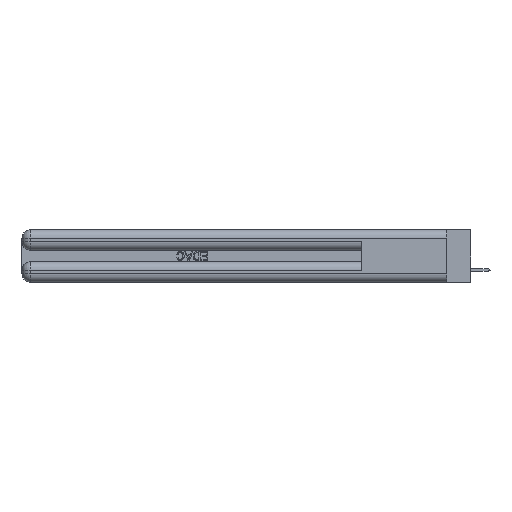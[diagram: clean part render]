
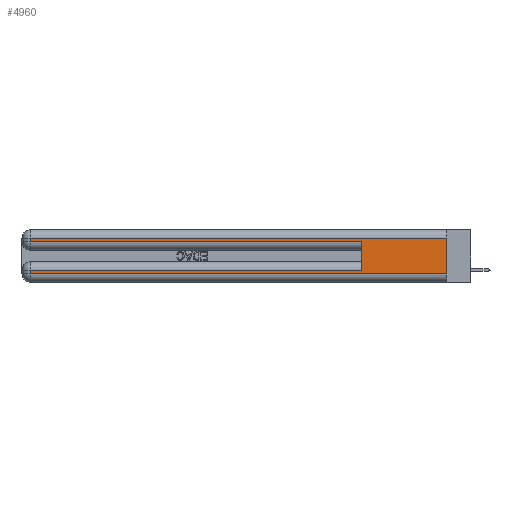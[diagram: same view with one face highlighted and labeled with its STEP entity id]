
A CAD part, left-side view. The second image highlights one B-rep face of the part: STEP entity #4960.
In plain terms, the highlighted planar face has unit normal (-1, 0, 0).
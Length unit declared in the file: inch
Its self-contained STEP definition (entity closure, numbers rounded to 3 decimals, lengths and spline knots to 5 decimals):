
#473 = CARTESIAN_POINT ( 'NONE',  ( 0., 0., 0.06 ) ) ;
#1075 = CARTESIAN_POINT ( 'NONE',  ( 0., 2.94, 0.085 ) ) ;
#2310 = LINE ( 'NONE', #2658, #29641 ) ;
#2658 = CARTESIAN_POINT ( 'NONE',  ( 0., 0., 0.37 ) ) ;
#2965 = VECTOR ( 'NONE', #22374, 39.37008 ) ;
#3176 = DIRECTION ( 'NONE',  ( 0., 1., 0. ) ) ;
#3217 = EDGE_CURVE ( 'NONE', #30540, #34532, #19578, .T. ) ;
#3498 = DIRECTION ( 'NONE',  ( 0., 0., -1. ) ) ;
#3556 = DIRECTION ( 'NONE',  ( 0., -1., 0. ) ) ;
#3927 = EDGE_CURVE ( 'NONE', #9854, #8282, #10133, .T. ) ;
#4305 = VECTOR ( 'NONE', #13085, 39.37008 ) ;
#4335 = CARTESIAN_POINT ( 'NONE',  ( 0., 2.94, 0.31 ) ) ;
#4768 = VECTOR ( 'NONE', #3498, 39.37008 ) ;
#4960 = ADVANCED_FACE ( 'NONE', ( #30598 ), #27456, .F. ) ;
#5708 = AXIS2_PLACEMENT_3D ( 'NONE', #32640, #30239, #32814 ) ;
#6026 = LINE ( 'NONE', #11940, #22527 ) ;
#6151 = DIRECTION ( 'NONE',  ( 0., -1., 0. ) ) ;
#6401 = DIRECTION ( 'NONE',  ( 0., 0., -1. ) ) ;
#8282 = VERTEX_POINT ( 'NONE', #4335 ) ;
#8548 = EDGE_CURVE ( 'NONE', #30540, #30297, #11151, .T. ) ;
#9031 = CARTESIAN_POINT ( 'NONE',  ( 0., 2.94, 0.285 ) ) ;
#9403 = LINE ( 'NONE', #17874, #4768 ) ;
#9787 = CARTESIAN_POINT ( 'NONE',  ( 0., 0.6, 0.285 ) ) ;
#9854 = VERTEX_POINT ( 'NONE', #11250 ) ;
#9961 = CARTESIAN_POINT ( 'NONE',  ( 0., 0., 0.31 ) ) ;
#10133 = LINE ( 'NONE', #9961, #4305 ) ;
#10393 = EDGE_CURVE ( 'NONE', #8282, #22889, #6026, .T. ) ;
#11151 = LINE ( 'NONE', #19776, #2965 ) ;
#11250 = CARTESIAN_POINT ( 'NONE',  ( 0., 0., 0.31 ) ) ;
#11940 = CARTESIAN_POINT ( 'NONE',  ( 0., 2.94, 0.37 ) ) ;
#12841 = ORIENTED_EDGE ( 'NONE', *, *, #3927, .T. ) ;
#13045 = ORIENTED_EDGE ( 'NONE', *, *, #20273, .T. ) ;
#13085 = DIRECTION ( 'NONE',  ( 0., 1., 0. ) ) ;
#15127 = EDGE_LOOP ( 'NONE', ( #30918, #12841, #17424, #26442, #24267, #24558, #13045, #35373 ) ) ;
#17424 = ORIENTED_EDGE ( 'NONE', *, *, #10393, .T. ) ;
#17874 = CARTESIAN_POINT ( 'NONE',  ( 0., 2.94, 0.37 ) ) ;
#18519 = VECTOR ( 'NONE', #3556, 39.37008 ) ;
#19578 = LINE ( 'NONE', #25851, #26596 ) ;
#19776 = CARTESIAN_POINT ( 'NONE',  ( 0., 0.6, 0.145 ) ) ;
#20273 = EDGE_CURVE ( 'NONE', #34532, #21901, #9403, .T. ) ;
#20800 = EDGE_CURVE ( 'NONE', #22889, #30297, #22375, .T. ) ;
#21901 = VERTEX_POINT ( 'NONE', #30898 ) ;
#21994 = DIRECTION ( 'NONE',  ( 0., 0., -1. ) ) ;
#22374 = DIRECTION ( 'NONE',  ( 0., 0., 1. ) ) ;
#22375 = LINE ( 'NONE', #25887, #22425 ) ;
#22425 = VECTOR ( 'NONE', #6151, 39.37008 ) ;
#22527 = VECTOR ( 'NONE', #6401, 39.37008 ) ;
#22889 = VERTEX_POINT ( 'NONE', #9031 ) ;
#23237 = CARTESIAN_POINT ( 'NONE',  ( 0., 0., 0.06 ) ) ;
#24267 = ORIENTED_EDGE ( 'NONE', *, *, #8548, .F. ) ;
#24558 = ORIENTED_EDGE ( 'NONE', *, *, #3217, .T. ) ;
#25035 = EDGE_CURVE ( 'NONE', #21901, #30119, #31233, .T. ) ;
#25851 = CARTESIAN_POINT ( 'NONE',  ( 0., 0., 0.085 ) ) ;
#25887 = CARTESIAN_POINT ( 'NONE',  ( 0., 0., 0.285 ) ) ;
#26442 = ORIENTED_EDGE ( 'NONE', *, *, #20800, .T. ) ;
#26596 = VECTOR ( 'NONE', #3176, 39.37008 ) ;
#27456 = PLANE ( 'NONE',  #5708 ) ;
#29516 = EDGE_CURVE ( 'NONE', #9854, #30119, #2310, .T. ) ;
#29641 = VECTOR ( 'NONE', #21994, 39.37008 ) ;
#30119 = VERTEX_POINT ( 'NONE', #23237 ) ;
#30239 = DIRECTION ( 'NONE',  ( 1., 0., 0. ) ) ;
#30297 = VERTEX_POINT ( 'NONE', #9787 ) ;
#30540 = VERTEX_POINT ( 'NONE', #35929 ) ;
#30598 = FACE_OUTER_BOUND ( 'NONE', #15127, .T. ) ;
#30898 = CARTESIAN_POINT ( 'NONE',  ( 0., 2.94, 0.06 ) ) ;
#30918 = ORIENTED_EDGE ( 'NONE', *, *, #29516, .F. ) ;
#31233 = LINE ( 'NONE', #473, #18519 ) ;
#32640 = CARTESIAN_POINT ( 'NONE',  ( 0., 0., 0.37 ) ) ;
#32814 = DIRECTION ( 'NONE',  ( 0., 0., -1. ) ) ;
#34532 = VERTEX_POINT ( 'NONE', #1075 ) ;
#35373 = ORIENTED_EDGE ( 'NONE', *, *, #25035, .T. ) ;
#35929 = CARTESIAN_POINT ( 'NONE',  ( 0., 0.6, 0.085 ) ) ;
